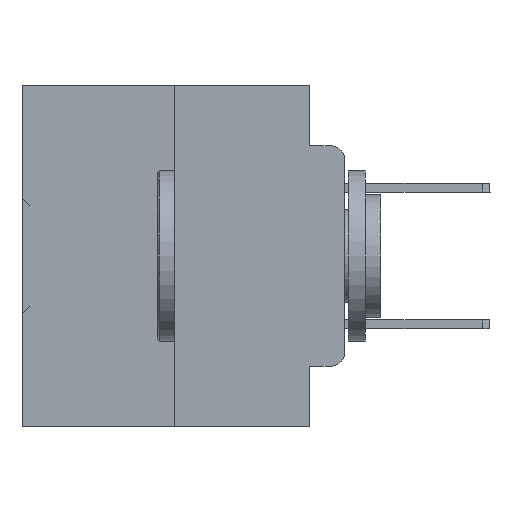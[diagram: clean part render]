
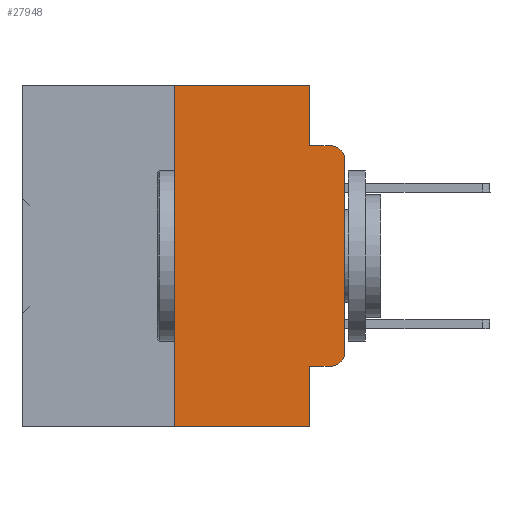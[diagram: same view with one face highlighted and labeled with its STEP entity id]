
A CAD part, left-side view. The second image highlights one B-rep face of the part: STEP entity #27948.
In plain terms, the highlighted planar face has unit normal (-1, 0, 0).
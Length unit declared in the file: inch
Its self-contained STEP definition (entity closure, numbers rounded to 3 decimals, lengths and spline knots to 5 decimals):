
#257 = CARTESIAN_POINT ( 'NONE',  ( 0., 0., -0.3915 ) ) ;
#508 = VECTOR ( 'NONE', #17948, 39.37008 ) ;
#552 = VERTEX_POINT ( 'NONE', #20877 ) ;
#961 = CIRCLE ( 'NONE', #14267, 0.02 ) ;
#3298 = VECTOR ( 'NONE', #27264, 39.37008 ) ;
#3415 = CIRCLE ( 'NONE', #7866, 0.02 ) ;
#4163 = VECTOR ( 'NONE', #25564, 39.37008 ) ;
#5225 = VECTOR ( 'NONE', #36613, 39.37008 ) ;
#5818 = ORIENTED_EDGE ( 'NONE', *, *, #6046, .T. ) ;
#5945 = ORIENTED_EDGE ( 'NONE', *, *, #10569, .T. ) ;
#5970 = VERTEX_POINT ( 'NONE', #11030 ) ;
#6046 = EDGE_CURVE ( 'NONE', #25888, #552, #26881, .T. ) ;
#6066 = DIRECTION ( 'NONE',  ( -1., 0., 0. ) ) ;
#6073 = FACE_OUTER_BOUND ( 'NONE', #28642, .T. ) ;
#6365 = DIRECTION ( 'NONE',  ( 0., 0., -1. ) ) ;
#6967 = EDGE_CURVE ( 'NONE', #32098, #9697, #9669, .T. ) ;
#7142 = CARTESIAN_POINT ( 'NONE',  ( 0., 0.02, -0.4115 ) ) ;
#7233 = CARTESIAN_POINT ( 'NONE',  ( 0., 0.051, -0.0885 ) ) ;
#7866 = AXIS2_PLACEMENT_3D ( 'NONE', #9723, #18857, #6365 ) ;
#8850 = DIRECTION ( 'NONE',  ( 1., 0., 0. ) ) ;
#9039 = PLANE ( 'NONE',  #15920 ) ;
#9469 = EDGE_CURVE ( 'NONE', #29017, #5970, #961, .T. ) ;
#9618 = DIRECTION ( 'NONE',  ( 0., 0., -1. ) ) ;
#9669 = LINE ( 'NONE', #36247, #29222 ) ;
#9681 = CARTESIAN_POINT ( 'NONE',  ( 0., 0.051, -0.4115 ) ) ;
#9682 = CARTESIAN_POINT ( 'NONE',  ( 0., 0.25, 0. ) ) ;
#9697 = VERTEX_POINT ( 'NONE', #7233 ) ;
#9723 = CARTESIAN_POINT ( 'NONE',  ( 0., 0.02, -0.3915 ) ) ;
#10234 = ORIENTED_EDGE ( 'NONE', *, *, #37597, .T. ) ;
#10569 = EDGE_CURVE ( 'NONE', #34515, #29017, #27954, .T. ) ;
#10725 = ORIENTED_EDGE ( 'NONE', *, *, #9469, .T. ) ;
#10994 = CARTESIAN_POINT ( 'NONE',  ( 0., 0.051, 0. ) ) ;
#11030 = CARTESIAN_POINT ( 'NONE',  ( 0., 0.02, -0.0885 ) ) ;
#12029 = LINE ( 'NONE', #36024, #5225 ) ;
#12205 = CARTESIAN_POINT ( 'NONE',  ( 0., 0.473, 0. ) ) ;
#12285 = VECTOR ( 'NONE', #21999, 39.37008 ) ;
#12912 = EDGE_CURVE ( 'NONE', #16930, #32098, #22720, .T. ) ;
#13812 = DIRECTION ( 'NONE',  ( 0., -1., 0. ) ) ;
#14267 = AXIS2_PLACEMENT_3D ( 'NONE', #15192, #6066, #9618 ) ;
#15192 = CARTESIAN_POINT ( 'NONE',  ( 0., 0.02, -0.1085 ) ) ;
#15920 = AXIS2_PLACEMENT_3D ( 'NONE', #12205, #8850, #30854 ) ;
#16930 = VERTEX_POINT ( 'NONE', #25485 ) ;
#17243 = ORIENTED_EDGE ( 'NONE', *, *, #18929, .T. ) ;
#17948 = DIRECTION ( 'NONE',  ( 0., -1., 0. ) ) ;
#18537 = CARTESIAN_POINT ( 'NONE',  ( 0., 0.473, -0.5 ) ) ;
#18857 = DIRECTION ( 'NONE',  ( -1., 0., 0. ) ) ;
#18929 = EDGE_CURVE ( 'NONE', #28910, #28706, #32642, .T. ) ;
#19074 = VECTOR ( 'NONE', #28678, 39.37008 ) ;
#19759 = LINE ( 'NONE', #26309, #19074 ) ;
#20754 = CARTESIAN_POINT ( 'NONE',  ( 0., 0.051, -0.4115 ) ) ;
#20877 = CARTESIAN_POINT ( 'NONE',  ( 0., 0.051, -0.5 ) ) ;
#21999 = DIRECTION ( 'NONE',  ( 0., 0., 1. ) ) ;
#22618 = CARTESIAN_POINT ( 'NONE',  ( 0., 0., 0. ) ) ;
#22720 = LINE ( 'NONE', #34802, #31936 ) ;
#22774 = ORIENTED_EDGE ( 'NONE', *, *, #30566, .F. ) ;
#24362 = LINE ( 'NONE', #9682, #12285 ) ;
#25485 = CARTESIAN_POINT ( 'NONE',  ( 0., 0.25, 0. ) ) ;
#25564 = DIRECTION ( 'NONE',  ( 0., 0., 1. ) ) ;
#25888 = VERTEX_POINT ( 'NONE', #28029 ) ;
#26309 = CARTESIAN_POINT ( 'NONE',  ( 0., 0.051, 0. ) ) ;
#26881 = LINE ( 'NONE', #18537, #3298 ) ;
#27264 = DIRECTION ( 'NONE',  ( 0., -1., 0. ) ) ;
#27385 = ORIENTED_EDGE ( 'NONE', *, *, #37962, .F. ) ;
#27533 = CARTESIAN_POINT ( 'NONE',  ( 0., 0., -0.1085 ) ) ;
#27948 = ADVANCED_FACE ( 'NONE', ( #6073 ), #9039, .F. ) ;
#27954 = LINE ( 'NONE', #22618, #4163 ) ;
#28029 = CARTESIAN_POINT ( 'NONE',  ( 0., 0.25, -0.5 ) ) ;
#28642 = EDGE_LOOP ( 'NONE', ( #5945, #10725, #30875, #28817, #33043, #27385, #5818, #22774, #17243, #10234 ) ) ;
#28678 = DIRECTION ( 'NONE',  ( 0., 0., -1. ) ) ;
#28706 = VERTEX_POINT ( 'NONE', #7142 ) ;
#28817 = ORIENTED_EDGE ( 'NONE', *, *, #6967, .F. ) ;
#28910 = VERTEX_POINT ( 'NONE', #9681 ) ;
#29017 = VERTEX_POINT ( 'NONE', #27533 ) ;
#29222 = VECTOR ( 'NONE', #30482, 39.37008 ) ;
#30482 = DIRECTION ( 'NONE',  ( 0., 0., -1. ) ) ;
#30566 = EDGE_CURVE ( 'NONE', #28910, #552, #19759, .T. ) ;
#30854 = DIRECTION ( 'NONE',  ( 0., 0., -1. ) ) ;
#30875 = ORIENTED_EDGE ( 'NONE', *, *, #33049, .F. ) ;
#31936 = VECTOR ( 'NONE', #13812, 39.37008 ) ;
#32098 = VERTEX_POINT ( 'NONE', #10994 ) ;
#32642 = LINE ( 'NONE', #20754, #508 ) ;
#33043 = ORIENTED_EDGE ( 'NONE', *, *, #12912, .F. ) ;
#33049 = EDGE_CURVE ( 'NONE', #9697, #5970, #12029, .T. ) ;
#34515 = VERTEX_POINT ( 'NONE', #257 ) ;
#34802 = CARTESIAN_POINT ( 'NONE',  ( 0., 0.473, 0. ) ) ;
#36024 = CARTESIAN_POINT ( 'NONE',  ( 0., 0.051, -0.0885 ) ) ;
#36247 = CARTESIAN_POINT ( 'NONE',  ( 0., 0.051, 0. ) ) ;
#36613 = DIRECTION ( 'NONE',  ( 0., -1., 0. ) ) ;
#37597 = EDGE_CURVE ( 'NONE', #28706, #34515, #3415, .T. ) ;
#37962 = EDGE_CURVE ( 'NONE', #25888, #16930, #24362, .T. ) ;
